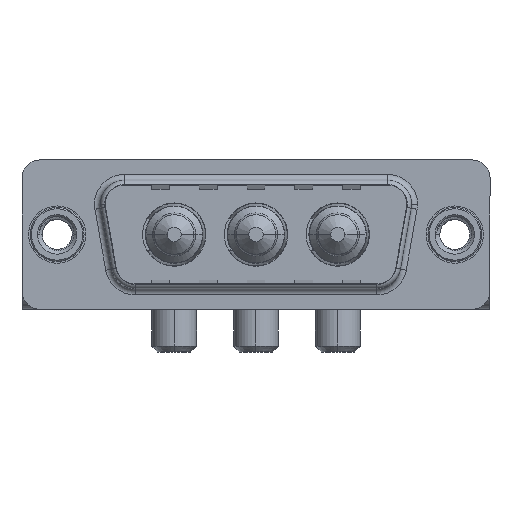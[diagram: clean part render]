
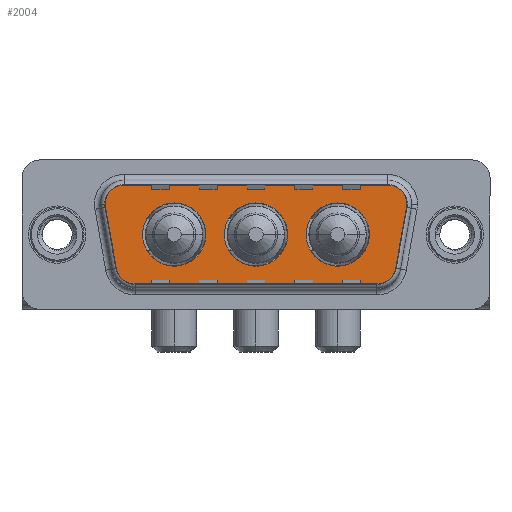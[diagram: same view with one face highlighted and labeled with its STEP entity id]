
A CAD part, top view. The second image highlights one B-rep face of the part: STEP entity #2004.
In plain terms, the highlighted planar face has unit normal (0, 0, 1).
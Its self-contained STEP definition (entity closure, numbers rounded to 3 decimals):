
#89 = EDGE_CURVE ( 'NONE', #10024, #9968, #10643, .T. ) ;
#383 = DIRECTION ( 'NONE',  ( 0., 0., 1. ) ) ;
#439 = CARTESIAN_POINT ( 'NONE',  ( 6.434, -4.9, 0. ) ) ;
#452 = EDGE_LOOP ( 'NONE', ( #7581, #11668 ) ) ;
#459 = AXIS2_PLACEMENT_3D ( 'NONE', #8769, #9876, #8533 ) ;
#742 = CARTESIAN_POINT ( 'NONE',  ( 5.411, 2.9, 0. ) ) ;
#776 = CARTESIAN_POINT ( 'NONE',  ( 14., 0., 0. ) ) ;
#911 = CIRCLE ( 'NONE', #10620, 2.65 ) ;
#920 = AXIS2_PLACEMENT_3D ( 'NONE', #13535, #7634, #4132 ) ;
#992 = VERTEX_POINT ( 'NONE', #12044 ) ;
#1057 = CARTESIAN_POINT ( 'NONE',  ( 12.45, 0., 0. ) ) ;
#1334 = CIRCLE ( 'NONE', #3083, 2.65 ) ;
#1379 = AXIS2_PLACEMENT_3D ( 'NONE', #4438, #11452, #9108 ) ;
#1431 = CARTESIAN_POINT ( 'NONE',  ( 6.434, -4.9, 0. ) ) ;
#1502 = CARTESIAN_POINT ( 'NONE',  ( 29.889, 2.9, 0. ) ) ;
#1564 = DIRECTION ( 'NONE',  ( 0., 0., 1. ) ) ;
#1566 = CARTESIAN_POINT ( 'NONE',  ( 4.464, -3.247, 0. ) ) ;
#1572 = ORIENTED_EDGE ( 'NONE', *, *, #89, .T. ) ;
#1589 = LINE ( 'NONE', #13417, #3219 ) ;
#1714 = CARTESIAN_POINT ( 'NONE',  ( 16.65, 0., 0. ) ) ;
#1759 = CIRCLE ( 'NONE', #7483, 2. ) ;
#1770 = ORIENTED_EDGE ( 'NONE', *, *, #6469, .T. ) ;
#1877 = EDGE_CURVE ( 'NONE', #5337, #2565, #1334, .T. ) ;
#1921 = DIRECTION ( 'NONE',  ( 1., 0., 0. ) ) ;
#2004 = ADVANCED_FACE ( 'NONE', ( #4931, #12080, #4707, #5804 ), #12947, .T. ) ;
#2148 = VERTEX_POINT ( 'NONE', #15056 ) ;
#2381 = ORIENTED_EDGE ( 'NONE', *, *, #12257, .T. ) ;
#2389 = CARTESIAN_POINT ( 'NONE',  ( 26.15, 0., 0. ) ) ;
#2489 = EDGE_CURVE ( 'NONE', #6935, #5979, #2809, .T. ) ;
#2565 = VERTEX_POINT ( 'NONE', #9745 ) ;
#2754 = EDGE_CURVE ( 'NONE', #2148, #5476, #14730, .T. ) ;
#2809 = CIRCLE ( 'NONE', #12501, 2.65 ) ;
#3083 = AXIS2_PLACEMENT_3D ( 'NONE', #11934, #10548, #7271 ) ;
#3112 = ORIENTED_EDGE ( 'NONE', *, *, #12258, .F. ) ;
#3175 = DIRECTION ( 'NONE',  ( -1., 0., 0. ) ) ;
#3219 = VECTOR ( 'NONE', #6135, 1000. ) ;
#3538 = ORIENTED_EDGE ( 'NONE', *, *, #12278, .T. ) ;
#3693 = AXIS2_PLACEMENT_3D ( 'NONE', #5077, #1564, #5156 ) ;
#3806 = ORIENTED_EDGE ( 'NONE', *, *, #14370, .T. ) ;
#3897 = DIRECTION ( 'NONE',  ( 1., 0., 0. ) ) ;
#3945 = CIRCLE ( 'NONE', #13881, 2.65 ) ;
#4132 = DIRECTION ( 'NONE',  ( -1., 0., 0. ) ) ;
#4438 = CARTESIAN_POINT ( 'NONE',  ( 9.8, 0., 0. ) ) ;
#4527 = CARTESIAN_POINT ( 'NONE',  ( 29.859, 2.553, 0. ) ) ;
#4530 = VERTEX_POINT ( 'NONE', #11849 ) ;
#4548 = DIRECTION ( 'NONE',  ( 0., 0., 1. ) ) ;
#4707 = FACE_BOUND ( 'NONE', #452, .T. ) ;
#4931 = FACE_BOUND ( 'NONE', #11311, .T. ) ;
#5077 = CARTESIAN_POINT ( 'NONE',  ( 26.866, -2.9, 0. ) ) ;
#5156 = DIRECTION ( 'NONE',  ( 1., 0., 0. ) ) ;
#5337 = VERTEX_POINT ( 'NONE', #2389 ) ;
#5346 = VECTOR ( 'NONE', #5785, 1000. ) ;
#5476 = VERTEX_POINT ( 'NONE', #1502 ) ;
#5785 = DIRECTION ( 'NONE',  ( 0.174, 0.985, 0. ) ) ;
#5804 = FACE_OUTER_BOUND ( 'NONE', #15251, .T. ) ;
#5843 = VERTEX_POINT ( 'NONE', #7342 ) ;
#5905 = DIRECTION ( 'NONE',  ( 0., 0., 1. ) ) ;
#5979 = VERTEX_POINT ( 'NONE', #8642 ) ;
#6048 = VERTEX_POINT ( 'NONE', #1566 ) ;
#6135 = DIRECTION ( 'NONE',  ( 0.174, -0.985, 0. ) ) ;
#6153 = LINE ( 'NONE', #439, #7188 ) ;
#6249 = DIRECTION ( 'NONE',  ( 0., 0., 1. ) ) ;
#6405 = CIRCLE ( 'NONE', #920, 2. ) ;
#6446 = CIRCLE ( 'NONE', #3693, 2. ) ;
#6469 = EDGE_CURVE ( 'NONE', #5843, #2148, #7881, .T. ) ;
#6513 = DIRECTION ( 'NONE',  ( 0., 0., 1. ) ) ;
#6864 = CIRCLE ( 'NONE', #1379, 2.65 ) ;
#6898 = CARTESIAN_POINT ( 'NONE',  ( 9.8, 0., 0. ) ) ;
#6935 = VERTEX_POINT ( 'NONE', #776 ) ;
#6967 = EDGE_CURVE ( 'NONE', #4530, #11179, #6864, .T. ) ;
#7188 = VECTOR ( 'NONE', #13208, 1000. ) ;
#7198 = DIRECTION ( 'NONE',  ( 1., 0., 0. ) ) ;
#7271 = DIRECTION ( 'NONE',  ( 1., 0., 0. ) ) ;
#7342 = CARTESIAN_POINT ( 'NONE',  ( 28.836, -3.247, 0. ) ) ;
#7483 = AXIS2_PLACEMENT_3D ( 'NONE', #742, #6513, #1921 ) ;
#7581 = ORIENTED_EDGE ( 'NONE', *, *, #13052, .F. ) ;
#7634 = DIRECTION ( 'NONE',  ( 0., 0., 1. ) ) ;
#7683 = VERTEX_POINT ( 'NONE', #15306 ) ;
#7776 = ORIENTED_EDGE ( 'NONE', *, *, #8290, .F. ) ;
#7881 = LINE ( 'NONE', #4527, #5346 ) ;
#8203 = CARTESIAN_POINT ( 'NONE',  ( 26.866, -2.9, 0. ) ) ;
#8290 = EDGE_CURVE ( 'NONE', #5979, #6935, #911, .T. ) ;
#8533 = DIRECTION ( 'NONE',  ( -1., 0., 0. ) ) ;
#8642 = CARTESIAN_POINT ( 'NONE',  ( 19.3, 0., 0. ) ) ;
#8769 = CARTESIAN_POINT ( 'NONE',  ( 6.434, -2.9, 0. ) ) ;
#8775 = AXIS2_PLACEMENT_3D ( 'NONE', #11811, #5905, #3175 ) ;
#8837 = CARTESIAN_POINT ( 'NONE',  ( 27.889, 4.9, 0. ) ) ;
#8971 = EDGE_CURVE ( 'NONE', #5476, #10024, #6405, .T. ) ;
#9108 = DIRECTION ( 'NONE',  ( 1., 0., 0. ) ) ;
#9634 = CARTESIAN_POINT ( 'NONE',  ( 5.411, 4.9, 0. ) ) ;
#9745 = CARTESIAN_POINT ( 'NONE',  ( 20.85, 0., 0. ) ) ;
#9838 = ORIENTED_EDGE ( 'NONE', *, *, #1877, .F. ) ;
#9876 = DIRECTION ( 'NONE',  ( 0., 0., 1. ) ) ;
#9968 = VERTEX_POINT ( 'NONE', #9634 ) ;
#10024 = VERTEX_POINT ( 'NONE', #8837 ) ;
#10132 = DIRECTION ( 'NONE',  ( 1., 0., 0. ) ) ;
#10410 = EDGE_CURVE ( 'NONE', #992, #5843, #6446, .T. ) ;
#10428 = AXIS2_PLACEMENT_3D ( 'NONE', #8203, #14254, #7198 ) ;
#10548 = DIRECTION ( 'NONE',  ( 0., 0., 1. ) ) ;
#10620 = AXIS2_PLACEMENT_3D ( 'NONE', #1714, #383, #10132 ) ;
#10643 = LINE ( 'NONE', #15386, #15248 ) ;
#10714 = EDGE_LOOP ( 'NONE', ( #9838, #3112 ) ) ;
#10936 = CIRCLE ( 'NONE', #12165, 2.65 ) ;
#11033 = ORIENTED_EDGE ( 'NONE', *, *, #2754, .T. ) ;
#11179 = VERTEX_POINT ( 'NONE', #1057 ) ;
#11249 = ORIENTED_EDGE ( 'NONE', *, *, #8971, .T. ) ;
#11311 = EDGE_LOOP ( 'NONE', ( #7776, #14368 ) ) ;
#11452 = DIRECTION ( 'NONE',  ( 0., 0., 1. ) ) ;
#11614 = ORIENTED_EDGE ( 'NONE', *, *, #12731, .T. ) ;
#11638 = DIRECTION ( 'NONE',  ( 1., 0., 0. ) ) ;
#11668 = ORIENTED_EDGE ( 'NONE', *, *, #6967, .F. ) ;
#11811 = CARTESIAN_POINT ( 'NONE',  ( 27.889, 2.9, 0. ) ) ;
#11849 = CARTESIAN_POINT ( 'NONE',  ( 7.15, 0., 0. ) ) ;
#11934 = CARTESIAN_POINT ( 'NONE',  ( 23.5, 0., 0. ) ) ;
#11945 = VERTEX_POINT ( 'NONE', #1431 ) ;
#12044 = CARTESIAN_POINT ( 'NONE',  ( 26.866, -4.9, 0. ) ) ;
#12080 = FACE_BOUND ( 'NONE', #10714, .T. ) ;
#12165 = AXIS2_PLACEMENT_3D ( 'NONE', #6898, #4548, #11638 ) ;
#12194 = DIRECTION ( 'NONE',  ( 0., 0., 1. ) ) ;
#12257 = EDGE_CURVE ( 'NONE', #11945, #992, #6153, .T. ) ;
#12258 = EDGE_CURVE ( 'NONE', #2565, #5337, #3945, .T. ) ;
#12278 = EDGE_CURVE ( 'NONE', #6048, #11945, #12652, .T. ) ;
#12501 = AXIS2_PLACEMENT_3D ( 'NONE', #15353, #6249, #3897 ) ;
#12632 = ORIENTED_EDGE ( 'NONE', *, *, #10410, .T. ) ;
#12652 = CIRCLE ( 'NONE', #459, 2. ) ;
#12731 = EDGE_CURVE ( 'NONE', #7683, #6048, #1589, .T. ) ;
#12947 = PLANE ( 'NONE',  #10428 ) ;
#13052 = EDGE_CURVE ( 'NONE', #11179, #4530, #10936, .T. ) ;
#13208 = DIRECTION ( 'NONE',  ( 1., 0., 0. ) ) ;
#13417 = CARTESIAN_POINT ( 'NONE',  ( 3.441, 2.553, 0. ) ) ;
#13535 = CARTESIAN_POINT ( 'NONE',  ( 27.889, 2.9, 0. ) ) ;
#13881 = AXIS2_PLACEMENT_3D ( 'NONE', #14682, #12194, #14447 ) ;
#14254 = DIRECTION ( 'NONE',  ( 0., 0., 1. ) ) ;
#14273 = DIRECTION ( 'NONE',  ( -1., 0., 0. ) ) ;
#14368 = ORIENTED_EDGE ( 'NONE', *, *, #2489, .F. ) ;
#14370 = EDGE_CURVE ( 'NONE', #9968, #7683, #1759, .T. ) ;
#14447 = DIRECTION ( 'NONE',  ( 1., 0., 0. ) ) ;
#14682 = CARTESIAN_POINT ( 'NONE',  ( 23.5, 0., 0. ) ) ;
#14730 = CIRCLE ( 'NONE', #8775, 2. ) ;
#15056 = CARTESIAN_POINT ( 'NONE',  ( 29.859, 2.553, 0. ) ) ;
#15248 = VECTOR ( 'NONE', #14273, 1000. ) ;
#15251 = EDGE_LOOP ( 'NONE', ( #12632, #1770, #11033, #11249, #1572, #3806, #11614, #3538, #2381 ) ) ;
#15306 = CARTESIAN_POINT ( 'NONE',  ( 3.441, 2.553, 0. ) ) ;
#15353 = CARTESIAN_POINT ( 'NONE',  ( 16.65, 0., 0. ) ) ;
#15386 = CARTESIAN_POINT ( 'NONE',  ( 5.411, 4.9, 0. ) ) ;
